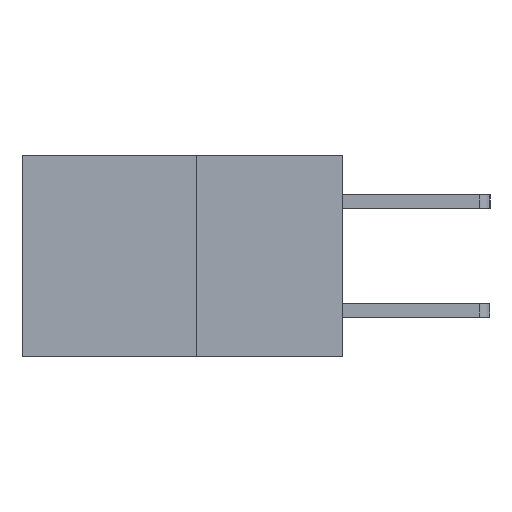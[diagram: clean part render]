
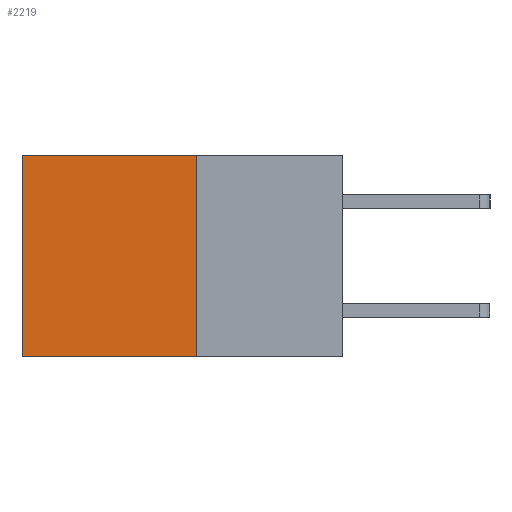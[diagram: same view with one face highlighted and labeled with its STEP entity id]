
A CAD part, left-side view. The second image highlights one B-rep face of the part: STEP entity #2219.
In plain terms, the highlighted planar face has unit normal (-1, 0, 0).
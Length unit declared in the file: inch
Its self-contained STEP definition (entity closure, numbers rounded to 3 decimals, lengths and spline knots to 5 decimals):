
#255 = VERTEX_POINT ( 'NONE', #1186 ) ;
#564 = EDGE_CURVE ( 'NONE', #5254, #255, #2554, .T. ) ;
#709 = VERTEX_POINT ( 'NONE', #8173 ) ;
#877 = DIRECTION ( 'NONE',  ( 0., 0., -1. ) ) ;
#1023 = DIRECTION ( 'NONE',  ( 0., 1., 0. ) ) ;
#1043 = DIRECTION ( 'NONE',  ( 1., 0., 0. ) ) ;
#1102 = CARTESIAN_POINT ( 'NONE',  ( 0.277, 0.59, 0. ) ) ;
#1186 = CARTESIAN_POINT ( 'NONE',  ( 0.277, 0.59, -0.37 ) ) ;
#1308 = LINE ( 'NONE', #3793, #3050 ) ;
#1775 = ORIENTED_EDGE ( 'NONE', *, *, #2327, .F. ) ;
#1995 = VERTEX_POINT ( 'NONE', #8835 ) ;
#2219 = ADVANCED_FACE ( 'NONE', ( #3066 ), #3321, .F. ) ;
#2327 = EDGE_CURVE ( 'NONE', #709, #1995, #7009, .T. ) ;
#2382 = CARTESIAN_POINT ( 'NONE',  ( 0.277, 0.27, 0. ) ) ;
#2540 = DIRECTION ( 'NONE',  ( 0., 1., 0. ) ) ;
#2554 = LINE ( 'NONE', #8388, #7789 ) ;
#3050 = VECTOR ( 'NONE', #1023, 39.37008 ) ;
#3066 = FACE_OUTER_BOUND ( 'NONE', #4446, .T. ) ;
#3255 = CARTESIAN_POINT ( 'NONE',  ( 0.277, 0.27, -0.37 ) ) ;
#3321 = PLANE ( 'NONE',  #3635 ) ;
#3365 = EDGE_CURVE ( 'NONE', #1995, #255, #1308, .T. ) ;
#3396 = VECTOR ( 'NONE', #5259, 39.37008 ) ;
#3635 = AXIS2_PLACEMENT_3D ( 'NONE', #3255, #1043, #877 ) ;
#3720 = ORIENTED_EDGE ( 'NONE', *, *, #4027, .T. ) ;
#3793 = CARTESIAN_POINT ( 'NONE',  ( 0.277, 0.27, -0.37 ) ) ;
#4027 = EDGE_CURVE ( 'NONE', #709, #5254, #6343, .T. ) ;
#4446 = EDGE_LOOP ( 'NONE', ( #7135, #8799, #1775, #3720 ) ) ;
#5084 = CARTESIAN_POINT ( 'NONE',  ( 0.277, 0.27, -0.37 ) ) ;
#5254 = VERTEX_POINT ( 'NONE', #1102 ) ;
#5259 = DIRECTION ( 'NONE',  ( 0., 0., -1. ) ) ;
#6129 = VECTOR ( 'NONE', #2540, 39.37008 ) ;
#6343 = LINE ( 'NONE', #2382, #6129 ) ;
#6443 = DIRECTION ( 'NONE',  ( 0., 0., -1. ) ) ;
#7009 = LINE ( 'NONE', #5084, #3396 ) ;
#7135 = ORIENTED_EDGE ( 'NONE', *, *, #564, .T. ) ;
#7789 = VECTOR ( 'NONE', #6443, 39.37008 ) ;
#8173 = CARTESIAN_POINT ( 'NONE',  ( 0.277, 0.27, 0. ) ) ;
#8388 = CARTESIAN_POINT ( 'NONE',  ( 0.277, 0.59, -0.37 ) ) ;
#8799 = ORIENTED_EDGE ( 'NONE', *, *, #3365, .F. ) ;
#8835 = CARTESIAN_POINT ( 'NONE',  ( 0.277, 0.27, -0.37 ) ) ;
